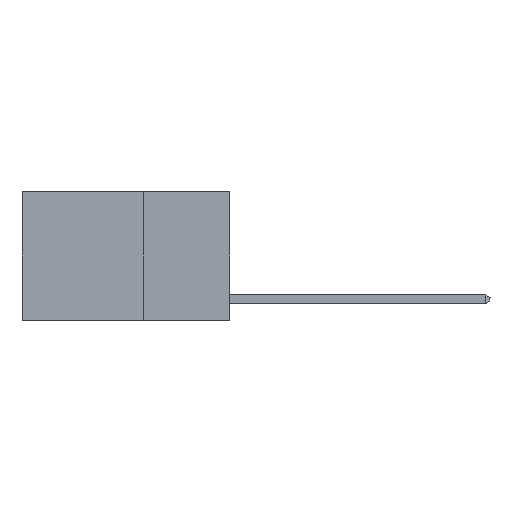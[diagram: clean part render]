
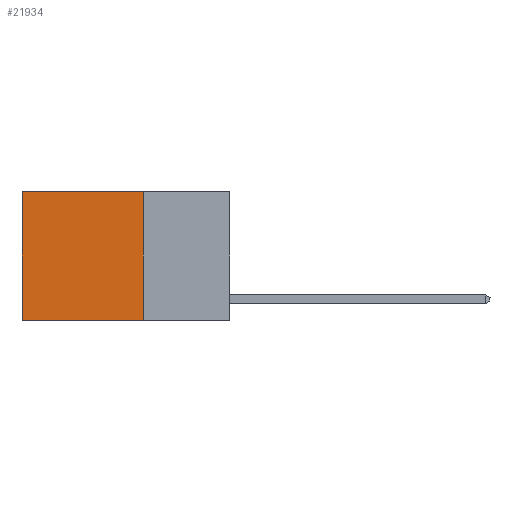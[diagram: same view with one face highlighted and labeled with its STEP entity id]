
A CAD part, left-side view. The second image highlights one B-rep face of the part: STEP entity #21934.
In plain terms, the highlighted planar face has unit normal (-1, 0, 0).
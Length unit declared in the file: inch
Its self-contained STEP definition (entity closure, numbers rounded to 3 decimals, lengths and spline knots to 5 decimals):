
#1699 = CARTESIAN_POINT ( 'NONE',  ( 0.2625, 0.6, 0. ) ) ;
#1868 = EDGE_LOOP ( 'NONE', ( #22854, #20452, #9228, #27849 ) ) ;
#2544 = EDGE_CURVE ( 'NONE', #14337, #24420, #15352, .T. ) ;
#3251 = CARTESIAN_POINT ( 'NONE',  ( 0.2625, 0.6, 0. ) ) ;
#4061 = EDGE_CURVE ( 'NONE', #7383, #22165, #24106, .T. ) ;
#5960 = DIRECTION ( 'NONE',  ( 0., 1., 0. ) ) ;
#6058 = DIRECTION ( 'NONE',  ( 1., 0., 0. ) ) ;
#6518 = CARTESIAN_POINT ( 'NONE',  ( 0.2625, 0.25, 0. ) ) ;
#7383 = VERTEX_POINT ( 'NONE', #1699 ) ;
#8679 = CARTESIAN_POINT ( 'NONE',  ( 0.2625, 0.25, -0.37 ) ) ;
#9228 = ORIENTED_EDGE ( 'NONE', *, *, #2544, .F. ) ;
#9857 = DIRECTION ( 'NONE',  ( 0., 1., 0. ) ) ;
#10150 = LINE ( 'NONE', #12116, #13779 ) ;
#10594 = DIRECTION ( 'NONE',  ( 0., 0., -1. ) ) ;
#12112 = VECTOR ( 'NONE', #5960, 39.37008 ) ;
#12116 = CARTESIAN_POINT ( 'NONE',  ( 0.2625, 0.25, 0. ) ) ;
#13263 = CARTESIAN_POINT ( 'NONE',  ( 0.2625, 0.25, -0.37 ) ) ;
#13779 = VECTOR ( 'NONE', #9857, 39.37008 ) ;
#13953 = EDGE_CURVE ( 'NONE', #24420, #22165, #17627, .T. ) ;
#14337 = VERTEX_POINT ( 'NONE', #28359 ) ;
#15352 = LINE ( 'NONE', #22639, #18318 ) ;
#17627 = LINE ( 'NONE', #8679, #12112 ) ;
#18076 = DIRECTION ( 'NONE',  ( 0., 0., -1. ) ) ;
#18318 = VECTOR ( 'NONE', #18076, 39.37008 ) ;
#19223 = CARTESIAN_POINT ( 'NONE',  ( 0.2625, 0.6, -0.37 ) ) ;
#19266 = DIRECTION ( 'NONE',  ( 0., 0., -1. ) ) ;
#20291 = PLANE ( 'NONE',  #23062 ) ;
#20452 = ORIENTED_EDGE ( 'NONE', *, *, #13953, .F. ) ;
#20453 = EDGE_CURVE ( 'NONE', #14337, #7383, #10150, .T. ) ;
#21934 = ADVANCED_FACE ( 'NONE', ( #29080 ), #20291, .F. ) ;
#22165 = VERTEX_POINT ( 'NONE', #19223 ) ;
#22639 = CARTESIAN_POINT ( 'NONE',  ( 0.2625, 0.25, 0. ) ) ;
#22854 = ORIENTED_EDGE ( 'NONE', *, *, #4061, .T. ) ;
#23062 = AXIS2_PLACEMENT_3D ( 'NONE', #6518, #6058, #10594 ) ;
#24106 = LINE ( 'NONE', #3251, #24775 ) ;
#24420 = VERTEX_POINT ( 'NONE', #13263 ) ;
#24775 = VECTOR ( 'NONE', #19266, 39.37008 ) ;
#27849 = ORIENTED_EDGE ( 'NONE', *, *, #20453, .T. ) ;
#28359 = CARTESIAN_POINT ( 'NONE',  ( 0.2625, 0.25, 0. ) ) ;
#29080 = FACE_OUTER_BOUND ( 'NONE', #1868, .T. ) ;
